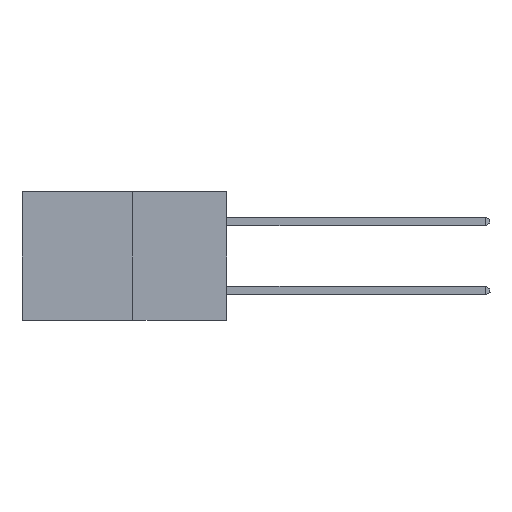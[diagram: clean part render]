
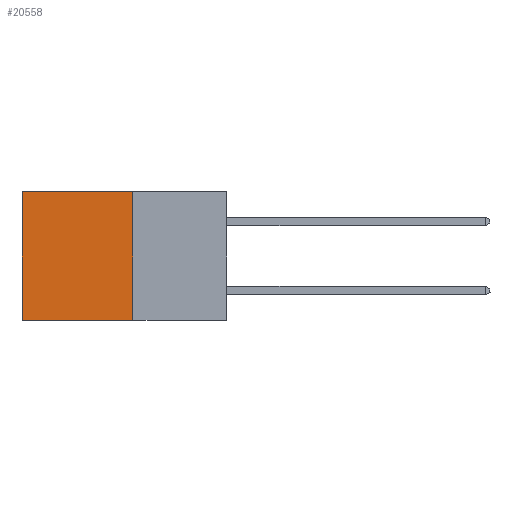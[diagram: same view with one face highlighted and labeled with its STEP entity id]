
A CAD part, left-side view. The second image highlights one B-rep face of the part: STEP entity #20558.
In plain terms, the highlighted planar face has unit normal (-1, 0, 0).
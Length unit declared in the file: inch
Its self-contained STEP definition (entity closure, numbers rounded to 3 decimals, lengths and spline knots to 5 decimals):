
#1275 = DIRECTION ( 'NONE',  ( 0., 0., -1. ) ) ;
#1784 = AXIS2_PLACEMENT_3D ( 'NONE', #25044, #13244, #1275 ) ;
#3127 = VERTEX_POINT ( 'NONE', #9946 ) ;
#3498 = ORIENTED_EDGE ( 'NONE', *, *, #23299, .T. ) ;
#3534 = LINE ( 'NONE', #10652, #8799 ) ;
#3687 = CARTESIAN_POINT ( 'NONE',  ( 0.277, 0.59, -0.37 ) ) ;
#4598 = FACE_OUTER_BOUND ( 'NONE', #17052, .T. ) ;
#4755 = VERTEX_POINT ( 'NONE', #3687 ) ;
#4989 = EDGE_CURVE ( 'NONE', #18566, #3127, #3534, .T. ) ;
#5408 = DIRECTION ( 'NONE',  ( 0., 0., -1. ) ) ;
#6192 = EDGE_CURVE ( 'NONE', #18566, #23831, #7507, .T. ) ;
#6501 = ORIENTED_EDGE ( 'NONE', *, *, #6192, .T. ) ;
#6882 = VECTOR ( 'NONE', #21653, 39.37008 ) ;
#7507 = LINE ( 'NONE', #21770, #6882 ) ;
#8799 = VECTOR ( 'NONE', #5408, 39.37008 ) ;
#9550 = ORIENTED_EDGE ( 'NONE', *, *, #4989, .F. ) ;
#9726 = VECTOR ( 'NONE', #24313, 39.37008 ) ;
#9901 = CARTESIAN_POINT ( 'NONE',  ( 0.277, 0.59, 0. ) ) ;
#9946 = CARTESIAN_POINT ( 'NONE',  ( 0.277, 0.27, -0.37 ) ) ;
#10652 = CARTESIAN_POINT ( 'NONE',  ( 0.277, 0.27, -0.37 ) ) ;
#11391 = CARTESIAN_POINT ( 'NONE',  ( 0.277, 0.27, -0.37 ) ) ;
#11886 = VECTOR ( 'NONE', #23228, 39.37008 ) ;
#13244 = DIRECTION ( 'NONE',  ( 1., 0., 0. ) ) ;
#15159 = PLANE ( 'NONE',  #1784 ) ;
#15957 = LINE ( 'NONE', #11391, #11886 ) ;
#17052 = EDGE_LOOP ( 'NONE', ( #3498, #20052, #9550, #6501 ) ) ;
#18566 = VERTEX_POINT ( 'NONE', #21558 ) ;
#20052 = ORIENTED_EDGE ( 'NONE', *, *, #24363, .F. ) ;
#20558 = ADVANCED_FACE ( 'NONE', ( #4598 ), #15159, .F. ) ;
#21558 = CARTESIAN_POINT ( 'NONE',  ( 0.277, 0.27, 0. ) ) ;
#21653 = DIRECTION ( 'NONE',  ( 0., 1., 0. ) ) ;
#21770 = CARTESIAN_POINT ( 'NONE',  ( 0.277, 0.27, 0. ) ) ;
#22334 = CARTESIAN_POINT ( 'NONE',  ( 0.277, 0.59, -0.37 ) ) ;
#23228 = DIRECTION ( 'NONE',  ( 0., 1., 0. ) ) ;
#23299 = EDGE_CURVE ( 'NONE', #23831, #4755, #25554, .T. ) ;
#23831 = VERTEX_POINT ( 'NONE', #9901 ) ;
#24313 = DIRECTION ( 'NONE',  ( 0., 0., -1. ) ) ;
#24363 = EDGE_CURVE ( 'NONE', #3127, #4755, #15957, .T. ) ;
#25044 = CARTESIAN_POINT ( 'NONE',  ( 0.277, 0.27, -0.37 ) ) ;
#25554 = LINE ( 'NONE', #22334, #9726 ) ;
